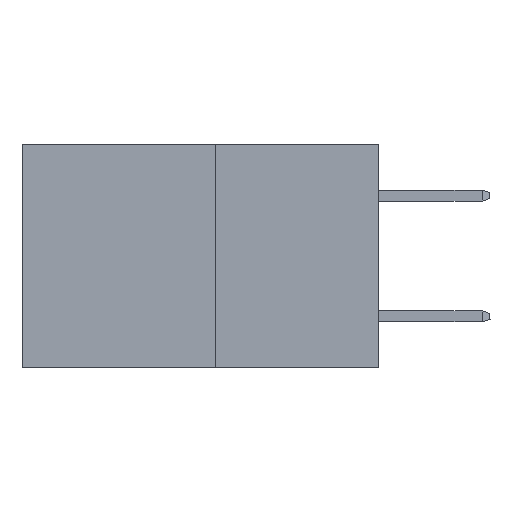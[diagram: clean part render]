
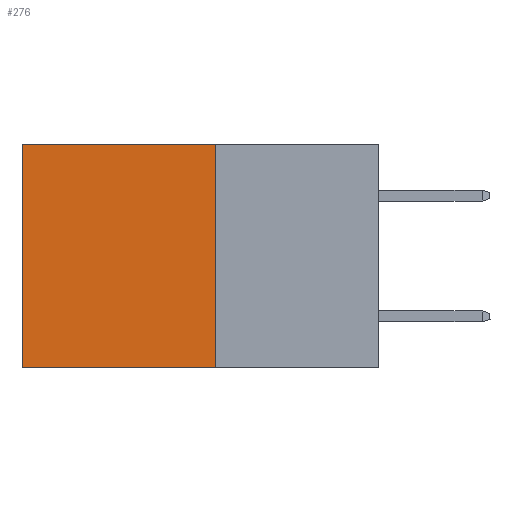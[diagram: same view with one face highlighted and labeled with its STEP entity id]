
A CAD part, left-side view. The second image highlights one B-rep face of the part: STEP entity #276.
In plain terms, the highlighted planar face has unit normal (-1, 0, 0).
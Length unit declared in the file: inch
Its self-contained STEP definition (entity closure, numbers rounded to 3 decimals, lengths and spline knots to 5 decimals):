
#60 = AXIS2_PLACEMENT_3D ( 'NONE', #4309, #4950, #4681 ) ;
#276 = ADVANCED_FACE ( 'NONE', ( #547 ), #1384, .F. ) ;
#547 = FACE_OUTER_BOUND ( 'NONE', #6703, .T. ) ;
#952 = LINE ( 'NONE', #10350, #12233 ) ;
#1384 = PLANE ( 'NONE',  #60 ) ;
#2092 = EDGE_CURVE ( 'NONE', #26435, #8483, #28476, .T. ) ;
#2339 = CARTESIAN_POINT ( 'NONE',  ( 0.277, 0.27, 0. ) ) ;
#2519 = DIRECTION ( 'NONE',  ( 0., 0., -1. ) ) ;
#4309 = CARTESIAN_POINT ( 'NONE',  ( 0.277, 0.27, -0.37 ) ) ;
#4681 = DIRECTION ( 'NONE',  ( 0., 0., -1. ) ) ;
#4950 = DIRECTION ( 'NONE',  ( 1., 0., 0. ) ) ;
#6623 = VERTEX_POINT ( 'NONE', #14421 ) ;
#6703 = EDGE_LOOP ( 'NONE', ( #26990, #24706, #17272, #10666 ) ) ;
#8087 = VERTEX_POINT ( 'NONE', #11880 ) ;
#8483 = VERTEX_POINT ( 'NONE', #17630 ) ;
#9619 = CARTESIAN_POINT ( 'NONE',  ( 0.277, 0.27, -0.37 ) ) ;
#10350 = CARTESIAN_POINT ( 'NONE',  ( 0.277, 0.59, -0.37 ) ) ;
#10666 = ORIENTED_EDGE ( 'NONE', *, *, #2092, .T. ) ;
#11523 = VECTOR ( 'NONE', #18491, 39.37008 ) ;
#11880 = CARTESIAN_POINT ( 'NONE',  ( 0.277, 0.27, -0.37 ) ) ;
#12233 = VECTOR ( 'NONE', #21517, 39.37008 ) ;
#12887 = LINE ( 'NONE', #18359, #18173 ) ;
#14421 = CARTESIAN_POINT ( 'NONE',  ( 0.277, 0.59, -0.37 ) ) ;
#17272 = ORIENTED_EDGE ( 'NONE', *, *, #28004, .F. ) ;
#17327 = DIRECTION ( 'NONE',  ( 0., 1., 0. ) ) ;
#17630 = CARTESIAN_POINT ( 'NONE',  ( 0.277, 0.59, 0. ) ) ;
#18173 = VECTOR ( 'NONE', #2519, 39.37008 ) ;
#18359 = CARTESIAN_POINT ( 'NONE',  ( 0.277, 0.27, -0.37 ) ) ;
#18491 = DIRECTION ( 'NONE',  ( 0., 1., 0. ) ) ;
#21517 = DIRECTION ( 'NONE',  ( 0., 0., -1. ) ) ;
#23417 = LINE ( 'NONE', #9619, #11523 ) ;
#24419 = EDGE_CURVE ( 'NONE', #8087, #6623, #23417, .T. ) ;
#24706 = ORIENTED_EDGE ( 'NONE', *, *, #24419, .F. ) ;
#26435 = VERTEX_POINT ( 'NONE', #28878 ) ;
#26990 = ORIENTED_EDGE ( 'NONE', *, *, #27626, .T. ) ;
#27626 = EDGE_CURVE ( 'NONE', #8483, #6623, #952, .T. ) ;
#27788 = VECTOR ( 'NONE', #17327, 39.37008 ) ;
#28004 = EDGE_CURVE ( 'NONE', #26435, #8087, #12887, .T. ) ;
#28476 = LINE ( 'NONE', #2339, #27788 ) ;
#28878 = CARTESIAN_POINT ( 'NONE',  ( 0.277, 0.27, 0. ) ) ;
